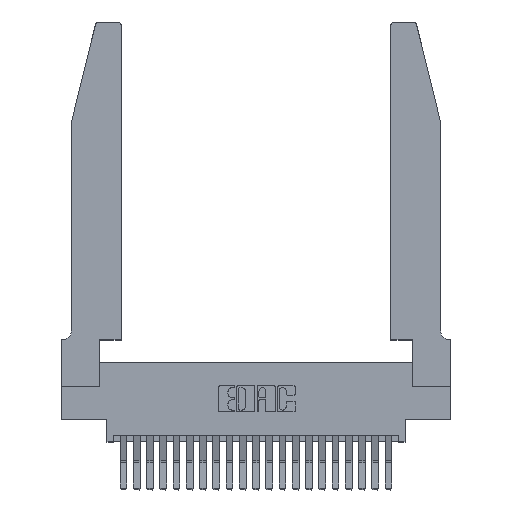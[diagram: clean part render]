
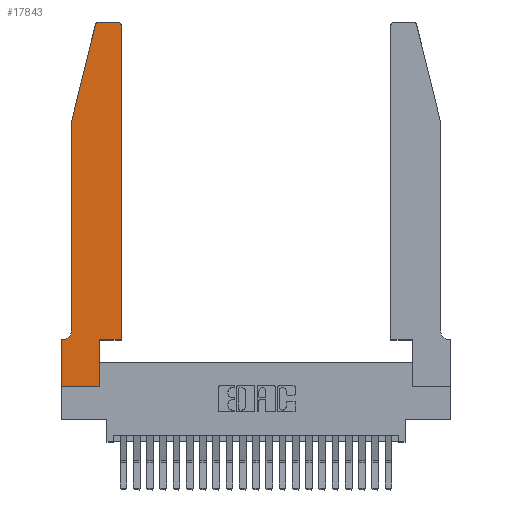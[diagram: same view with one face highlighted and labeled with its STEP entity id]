
A CAD part, top view. The second image highlights one B-rep face of the part: STEP entity #17843.
In plain terms, the highlighted planar face has unit normal (0, 0, 1).
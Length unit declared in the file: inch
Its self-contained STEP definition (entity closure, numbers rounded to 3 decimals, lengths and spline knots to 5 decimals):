
#11 = DIRECTION ( 'NONE',  ( -1., 0., 0. ) ) ;
#340 = CIRCLE ( 'NONE', #18576, 0.03 ) ;
#531 = DIRECTION ( 'NONE',  ( -1., 0., 0. ) ) ;
#863 = CARTESIAN_POINT ( 'NONE',  ( 0.0055, 0.42, 0.37 ) ) ;
#872 = VERTEX_POINT ( 'NONE', #18195 ) ;
#1419 = LINE ( 'NONE', #9031, #3202 ) ;
#1567 = VECTOR ( 'NONE', #8558, 39.37008 ) ;
#1706 = VERTEX_POINT ( 'NONE', #21522 ) ;
#1708 = VERTEX_POINT ( 'NONE', #4412 ) ;
#1736 = VERTEX_POINT ( 'NONE', #12627 ) ;
#1816 = CARTESIAN_POINT ( 'NONE',  ( 0.0755, 2., 0.37 ) ) ;
#2338 = LINE ( 'NONE', #22861, #19345 ) ;
#2446 = CARTESIAN_POINT ( 'NONE',  ( 0., 0.35, 0.37 ) ) ;
#2681 = ORIENTED_EDGE ( 'NONE', *, *, #3975, .T. ) ;
#2935 = VERTEX_POINT ( 'NONE', #1816 ) ;
#3202 = VECTOR ( 'NONE', #14683, 39.37008 ) ;
#3448 = VECTOR ( 'NONE', #24030, 39.37008 ) ;
#3975 = EDGE_CURVE ( 'NONE', #1736, #11189, #24037, .T. ) ;
#4296 = EDGE_CURVE ( 'NONE', #9362, #2935, #2338, .T. ) ;
#4412 = CARTESIAN_POINT ( 'NONE',  ( 0.2865, 0.35, 0.37 ) ) ;
#4452 = VECTOR ( 'NONE', #7939, 39.37008 ) ;
#4631 = FACE_OUTER_BOUND ( 'NONE', #7572, .T. ) ;
#4820 = EDGE_CURVE ( 'NONE', #11189, #17305, #9075, .T. ) ;
#5063 = EDGE_CURVE ( 'NONE', #1708, #7102, #1419, .T. ) ;
#5132 = ORIENTED_EDGE ( 'NONE', *, *, #21168, .T. ) ;
#5234 = VECTOR ( 'NONE', #11, 39.37008 ) ;
#5855 = CARTESIAN_POINT ( 'NONE',  ( 0.2865, 0.35, 0.37 ) ) ;
#6004 = EDGE_CURVE ( 'NONE', #20459, #1736, #17477, .T. ) ;
#6221 = CARTESIAN_POINT ( 'NONE',  ( 0., 0., 0.37 ) ) ;
#6346 = DIRECTION ( 'NONE',  ( 0., 0., 1. ) ) ;
#6431 = CARTESIAN_POINT ( 'NONE',  ( 0.4205, 2.72, 0.37 ) ) ;
#6585 = CARTESIAN_POINT ( 'NONE',  ( 0.0755, 2., 0.37 ) ) ;
#7102 = VERTEX_POINT ( 'NONE', #15575 ) ;
#7346 = VERTEX_POINT ( 'NONE', #12474 ) ;
#7572 = EDGE_LOOP ( 'NONE', ( #10460, #22051, #17089, #5132, #17737, #23774, #2681, #22592, #15823, #20421, #9714, #19372 ) ) ;
#7939 = DIRECTION ( 'NONE',  ( 0., -1., 0. ) ) ;
#8017 = CIRCLE ( 'NONE', #9020, 0.07 ) ;
#8152 = CARTESIAN_POINT ( 'NONE',  ( 0., 0., 0.37 ) ) ;
#8558 = DIRECTION ( 'NONE',  ( 0., -1., 0. ) ) ;
#9001 = CARTESIAN_POINT ( 'NONE',  ( 0.25487, 2.72718, 0.37 ) ) ;
#9020 = AXIS2_PLACEMENT_3D ( 'NONE', #863, #13946, #531 ) ;
#9031 = CARTESIAN_POINT ( 'NONE',  ( 0.4505, 0.35, 0.37 ) ) ;
#9075 = LINE ( 'NONE', #8152, #20218 ) ;
#9078 = CARTESIAN_POINT ( 'NONE',  ( 0.284, 2.72, 0.37 ) ) ;
#9333 = EDGE_CURVE ( 'NONE', #1706, #9362, #24087, .T. ) ;
#9362 = VERTEX_POINT ( 'NONE', #9001 ) ;
#9714 = ORIENTED_EDGE ( 'NONE', *, *, #23026, .T. ) ;
#10207 = DIRECTION ( 'NONE',  ( 1., 0., 0. ) ) ;
#10460 = ORIENTED_EDGE ( 'NONE', *, *, #17115, .T. ) ;
#10730 = EDGE_CURVE ( 'NONE', #18190, #7346, #340, .T. ) ;
#10937 = CARTESIAN_POINT ( 'NONE',  ( 0.0755, 0.35, 0.37 ) ) ;
#11189 = VERTEX_POINT ( 'NONE', #6221 ) ;
#11393 = CARTESIAN_POINT ( 'NONE',  ( 0., 0., 0.37 ) ) ;
#11668 = AXIS2_PLACEMENT_3D ( 'NONE', #9078, #18305, #20220 ) ;
#12474 = CARTESIAN_POINT ( 'NONE',  ( 0.4205, 2.75, 0.37 ) ) ;
#12566 = EDGE_CURVE ( 'NONE', #17305, #1708, #21072, .T. ) ;
#12627 = CARTESIAN_POINT ( 'NONE',  ( 0., 0.35, 0.37 ) ) ;
#13558 = LINE ( 'NONE', #14675, #23228 ) ;
#13656 = PLANE ( 'NONE',  #20571 ) ;
#13946 = DIRECTION ( 'NONE',  ( 0., 0., -1. ) ) ;
#14439 = DIRECTION ( 'NONE',  ( 0., 1., 0. ) ) ;
#14675 = CARTESIAN_POINT ( 'NONE',  ( 0.4505, 0.35, 0.37 ) ) ;
#14683 = DIRECTION ( 'NONE',  ( 1., 0., 0. ) ) ;
#15314 = LINE ( 'NONE', #6585, #1567 ) ;
#15575 = CARTESIAN_POINT ( 'NONE',  ( 0.4505, 0.35, 0.37 ) ) ;
#15823 = ORIENTED_EDGE ( 'NONE', *, *, #12566, .T. ) ;
#16527 = CARTESIAN_POINT ( 'NONE',  ( 0.2605, 2.75, 0.37 ) ) ;
#17089 = ORIENTED_EDGE ( 'NONE', *, *, #4296, .T. ) ;
#17095 = DIRECTION ( 'NONE',  ( -0.239, -0.971, 0. ) ) ;
#17115 = EDGE_CURVE ( 'NONE', #7346, #1706, #23099, .T. ) ;
#17305 = VERTEX_POINT ( 'NONE', #23771 ) ;
#17366 = DIRECTION ( 'NONE',  ( 0., 1., 0. ) ) ;
#17403 = CARTESIAN_POINT ( 'NONE',  ( 0.4505, 2.72, 0.37 ) ) ;
#17477 = LINE ( 'NONE', #10937, #3448 ) ;
#17737 = ORIENTED_EDGE ( 'NONE', *, *, #22204, .T. ) ;
#17843 = ADVANCED_FACE ( 'NONE', ( #4631 ), #13656, .T. ) ;
#18190 = VERTEX_POINT ( 'NONE', #17403 ) ;
#18195 = CARTESIAN_POINT ( 'NONE',  ( 0.0755, 0.42, 0.37 ) ) ;
#18305 = DIRECTION ( 'NONE',  ( 0., 0., 1. ) ) ;
#18576 = AXIS2_PLACEMENT_3D ( 'NONE', #6431, #6346, #10207 ) ;
#19330 = DIRECTION ( 'NONE',  ( 0., 0., 1. ) ) ;
#19345 = VECTOR ( 'NONE', #17095, 39.37008 ) ;
#19372 = ORIENTED_EDGE ( 'NONE', *, *, #10730, .T. ) ;
#19566 = CARTESIAN_POINT ( 'NONE',  ( 0.0055, 0.35, 0.37 ) ) ;
#20218 = VECTOR ( 'NONE', #21352, 39.37008 ) ;
#20220 = DIRECTION ( 'NONE',  ( 1., 0., 0. ) ) ;
#20421 = ORIENTED_EDGE ( 'NONE', *, *, #5063, .T. ) ;
#20459 = VERTEX_POINT ( 'NONE', #19566 ) ;
#20571 = AXIS2_PLACEMENT_3D ( 'NONE', #2446, #19330, #21331 ) ;
#21072 = LINE ( 'NONE', #5855, #21382 ) ;
#21168 = EDGE_CURVE ( 'NONE', #2935, #872, #15314, .T. ) ;
#21331 = DIRECTION ( 'NONE',  ( 1., 0., 0. ) ) ;
#21352 = DIRECTION ( 'NONE',  ( 1., 0., 0. ) ) ;
#21382 = VECTOR ( 'NONE', #17366, 39.37008 ) ;
#21522 = CARTESIAN_POINT ( 'NONE',  ( 0.284, 2.75, 0.37 ) ) ;
#22051 = ORIENTED_EDGE ( 'NONE', *, *, #9333, .T. ) ;
#22204 = EDGE_CURVE ( 'NONE', #872, #20459, #8017, .T. ) ;
#22592 = ORIENTED_EDGE ( 'NONE', *, *, #4820, .T. ) ;
#22861 = CARTESIAN_POINT ( 'NONE',  ( 0.0755, 2., 0.37 ) ) ;
#23026 = EDGE_CURVE ( 'NONE', #7102, #18190, #13558, .T. ) ;
#23099 = LINE ( 'NONE', #16527, #5234 ) ;
#23228 = VECTOR ( 'NONE', #14439, 39.37008 ) ;
#23771 = CARTESIAN_POINT ( 'NONE',  ( 0.2865, 0., 0.37 ) ) ;
#23774 = ORIENTED_EDGE ( 'NONE', *, *, #6004, .T. ) ;
#24030 = DIRECTION ( 'NONE',  ( -1., 0., 0. ) ) ;
#24037 = LINE ( 'NONE', #11393, #4452 ) ;
#24087 = CIRCLE ( 'NONE', #11668, 0.03 ) ;
